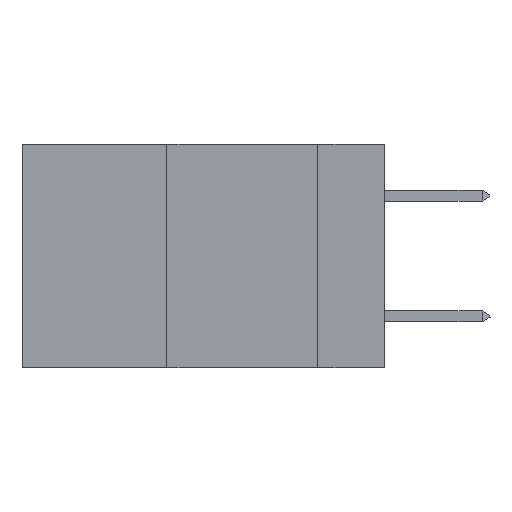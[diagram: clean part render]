
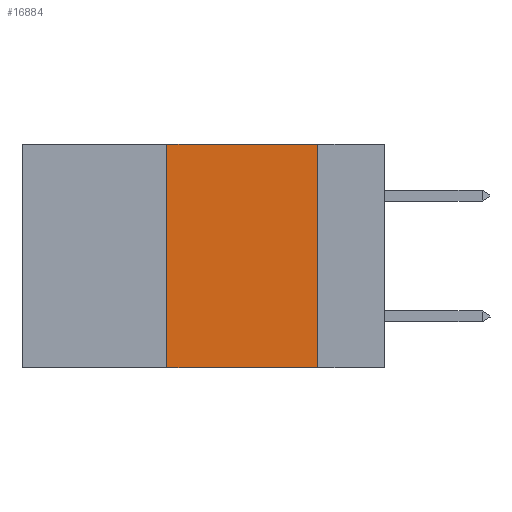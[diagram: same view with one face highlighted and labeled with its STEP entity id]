
A CAD part, left-side view. The second image highlights one B-rep face of the part: STEP entity #16884.
In plain terms, the highlighted planar face has unit normal (-1, 0, 0).
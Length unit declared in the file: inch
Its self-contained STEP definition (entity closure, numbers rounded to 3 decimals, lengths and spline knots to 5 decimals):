
#253 = VECTOR ( 'NONE', #7697, 39.37008 ) ;
#717 = PLANE ( 'NONE',  #11765 ) ;
#997 = LINE ( 'NONE', #1879, #14885 ) ;
#1621 = EDGE_CURVE ( 'NONE', #19189, #18592, #997, .T. ) ;
#1879 = CARTESIAN_POINT ( 'NONE',  ( 0., 0.11, 0. ) ) ;
#2141 = DIRECTION ( 'NONE',  ( 0., 0., -1. ) ) ;
#3152 = ORIENTED_EDGE ( 'NONE', *, *, #21576, .T. ) ;
#5116 = DIRECTION ( 'NONE',  ( 0., 0., 1. ) ) ;
#5167 = DIRECTION ( 'NONE',  ( 0., -1., 0. ) ) ;
#5845 = LINE ( 'NONE', #9589, #18146 ) ;
#7697 = DIRECTION ( 'NONE',  ( 0., -1., 0. ) ) ;
#7955 = ORIENTED_EDGE ( 'NONE', *, *, #9286, .F. ) ;
#9286 = EDGE_CURVE ( 'NONE', #9940, #19189, #26713, .T. ) ;
#9589 = CARTESIAN_POINT ( 'NONE',  ( 0., 0.36, 0. ) ) ;
#9940 = VERTEX_POINT ( 'NONE', #25498 ) ;
#11697 = ORIENTED_EDGE ( 'NONE', *, *, #13292, .F. ) ;
#11765 = AXIS2_PLACEMENT_3D ( 'NONE', #13029, #15152, #13200 ) ;
#12731 = CARTESIAN_POINT ( 'NONE',  ( 0., 0.11, -0.37 ) ) ;
#13029 = CARTESIAN_POINT ( 'NONE',  ( 0., 0.6, 0. ) ) ;
#13200 = DIRECTION ( 'NONE',  ( 0., 0., -1. ) ) ;
#13292 = EDGE_CURVE ( 'NONE', #19814, #9940, #5845, .T. ) ;
#13555 = LINE ( 'NONE', #19791, #16121 ) ;
#14885 = VECTOR ( 'NONE', #2141, 39.37008 ) ;
#15152 = DIRECTION ( 'NONE',  ( 1., 0., 0. ) ) ;
#16121 = VECTOR ( 'NONE', #5167, 39.37008 ) ;
#16884 = ADVANCED_FACE ( 'NONE', ( #17736 ), #717, .F. ) ;
#17736 = FACE_OUTER_BOUND ( 'NONE', #21726, .T. ) ;
#18146 = VECTOR ( 'NONE', #5116, 39.37008 ) ;
#18592 = VERTEX_POINT ( 'NONE', #12731 ) ;
#18789 = CARTESIAN_POINT ( 'NONE',  ( 0., 0.11, 0. ) ) ;
#19189 = VERTEX_POINT ( 'NONE', #18789 ) ;
#19791 = CARTESIAN_POINT ( 'NONE',  ( 0., 0.6, -0.37 ) ) ;
#19814 = VERTEX_POINT ( 'NONE', #24219 ) ;
#21576 = EDGE_CURVE ( 'NONE', #19814, #18592, #13555, .T. ) ;
#21726 = EDGE_LOOP ( 'NONE', ( #26443, #7955, #11697, #3152 ) ) ;
#24219 = CARTESIAN_POINT ( 'NONE',  ( 0., 0.36, -0.37 ) ) ;
#25498 = CARTESIAN_POINT ( 'NONE',  ( 0., 0.36, 0. ) ) ;
#26284 = CARTESIAN_POINT ( 'NONE',  ( 0., 0.6, 0. ) ) ;
#26443 = ORIENTED_EDGE ( 'NONE', *, *, #1621, .F. ) ;
#26713 = LINE ( 'NONE', #26284, #253 ) ;
